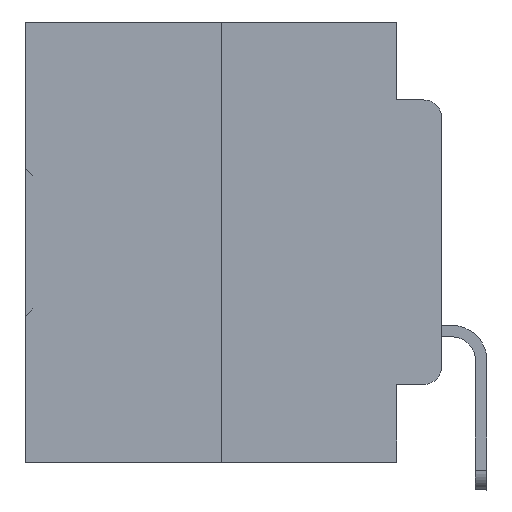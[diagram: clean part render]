
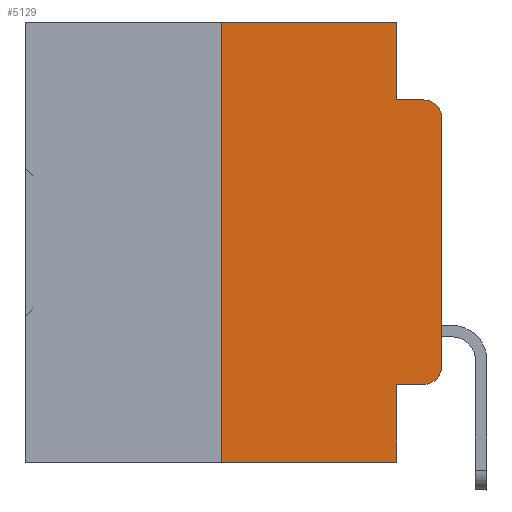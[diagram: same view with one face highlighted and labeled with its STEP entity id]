
A CAD part, left-side view. The second image highlights one B-rep face of the part: STEP entity #5129.
In plain terms, the highlighted planar face has unit normal (-1, 0, 0).
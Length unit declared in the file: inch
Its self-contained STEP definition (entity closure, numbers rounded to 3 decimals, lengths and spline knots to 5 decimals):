
#219 = DIRECTION ( 'NONE',  ( 1., 0., 0. ) ) ;
#1815 = CARTESIAN_POINT ( 'NONE',  ( 0., 0.02, -0.1085 ) ) ;
#3067 = VECTOR ( 'NONE', #6781, 39.37008 ) ;
#3185 = CARTESIAN_POINT ( 'NONE',  ( 0., 0.051, 0. ) ) ;
#3382 = DIRECTION ( 'NONE',  ( 0., 0., 1. ) ) ;
#3490 = CARTESIAN_POINT ( 'NONE',  ( 0., 0.25, 0. ) ) ;
#3536 = CARTESIAN_POINT ( 'NONE',  ( 0., 0., -0.3915 ) ) ;
#4029 = VERTEX_POINT ( 'NONE', #16849 ) ;
#4118 = VERTEX_POINT ( 'NONE', #9675 ) ;
#4264 = AXIS2_PLACEMENT_3D ( 'NONE', #32118, #4676, #4436 ) ;
#4436 = DIRECTION ( 'NONE',  ( 0., 0., -1. ) ) ;
#4676 = DIRECTION ( 'NONE',  ( -1., 0., 0. ) ) ;
#5129 = ADVANCED_FACE ( 'NONE', ( #27398 ), #30025, .F. ) ;
#5293 = EDGE_CURVE ( 'NONE', #20373, #29072, #19749, .T. ) ;
#5730 = DIRECTION ( 'NONE',  ( 0., 0., -1. ) ) ;
#6280 = CARTESIAN_POINT ( 'NONE',  ( 0., 0.051, -0.0885 ) ) ;
#6712 = EDGE_LOOP ( 'NONE', ( #7500, #19162, #9595, #32900, #20562, #15418, #29869, #10594, #18229, #23644 ) ) ;
#6781 = DIRECTION ( 'NONE',  ( 0., 0., 1. ) ) ;
#7350 = EDGE_CURVE ( 'NONE', #29072, #15682, #24922, .T. ) ;
#7380 = LINE ( 'NONE', #12807, #16774 ) ;
#7500 = ORIENTED_EDGE ( 'NONE', *, *, #5293, .T. ) ;
#7527 = DIRECTION ( 'NONE',  ( 0., 0., -1. ) ) ;
#8580 = VERTEX_POINT ( 'NONE', #26436 ) ;
#8662 = AXIS2_PLACEMENT_3D ( 'NONE', #19694, #219, #5730 ) ;
#9595 = ORIENTED_EDGE ( 'NONE', *, *, #26464, .F. ) ;
#9675 = CARTESIAN_POINT ( 'NONE',  ( 0., 0.02, -0.4115 ) ) ;
#9778 = LINE ( 'NONE', #3490, #32808 ) ;
#10130 = EDGE_CURVE ( 'NONE', #34146, #8580, #9778, .T. ) ;
#10342 = EDGE_CURVE ( 'NONE', #8580, #29618, #15295, .T. ) ;
#10594 = ORIENTED_EDGE ( 'NONE', *, *, #12152, .F. ) ;
#11087 = EDGE_CURVE ( 'NONE', #34146, #18029, #22066, .T. ) ;
#11795 = CARTESIAN_POINT ( 'NONE',  ( 0., 0., -0.1085 ) ) ;
#12152 = EDGE_CURVE ( 'NONE', #4029, #18029, #14723, .T. ) ;
#12328 = CARTESIAN_POINT ( 'NONE',  ( 0., 0.051, 0. ) ) ;
#12807 = CARTESIAN_POINT ( 'NONE',  ( 0., 0.051, -0.0885 ) ) ;
#14183 = AXIS2_PLACEMENT_3D ( 'NONE', #1815, #31512, #7527 ) ;
#14251 = VECTOR ( 'NONE', #14429, 39.37008 ) ;
#14429 = DIRECTION ( 'NONE',  ( 0., 0., -1. ) ) ;
#14723 = LINE ( 'NONE', #12328, #28371 ) ;
#14783 = VECTOR ( 'NONE', #18966, 39.37008 ) ;
#14804 = DIRECTION ( 'NONE',  ( 0., -1., 0. ) ) ;
#15295 = LINE ( 'NONE', #20558, #23442 ) ;
#15418 = ORIENTED_EDGE ( 'NONE', *, *, #10130, .F. ) ;
#15483 = EDGE_CURVE ( 'NONE', #4029, #4118, #30434, .T. ) ;
#15682 = VERTEX_POINT ( 'NONE', #31189 ) ;
#16466 = CARTESIAN_POINT ( 'NONE',  ( 0., 0.051, -0.5 ) ) ;
#16774 = VECTOR ( 'NONE', #23657, 39.37008 ) ;
#16849 = CARTESIAN_POINT ( 'NONE',  ( 0., 0.051, -0.4115 ) ) ;
#16979 = CARTESIAN_POINT ( 'NONE',  ( 0., 0.051, 0. ) ) ;
#18029 = VERTEX_POINT ( 'NONE', #16466 ) ;
#18131 = CARTESIAN_POINT ( 'NONE',  ( 0., 0.473, -0.5 ) ) ;
#18229 = ORIENTED_EDGE ( 'NONE', *, *, #15483, .T. ) ;
#18747 = VERTEX_POINT ( 'NONE', #6280 ) ;
#18831 = CARTESIAN_POINT ( 'NONE',  ( 0., 0.051, -0.4115 ) ) ;
#18966 = DIRECTION ( 'NONE',  ( 0., -1., 0. ) ) ;
#19162 = ORIENTED_EDGE ( 'NONE', *, *, #7350, .T. ) ;
#19694 = CARTESIAN_POINT ( 'NONE',  ( 0., 0.473, 0. ) ) ;
#19749 = LINE ( 'NONE', #28594, #3067 ) ;
#19797 = VECTOR ( 'NONE', #32768, 39.37008 ) ;
#20373 = VERTEX_POINT ( 'NONE', #3536 ) ;
#20558 = CARTESIAN_POINT ( 'NONE',  ( 0., 0.473, 0. ) ) ;
#20562 = ORIENTED_EDGE ( 'NONE', *, *, #10342, .F. ) ;
#22066 = LINE ( 'NONE', #18131, #14783 ) ;
#22387 = LINE ( 'NONE', #16979, #14251 ) ;
#23442 = VECTOR ( 'NONE', #14804, 39.37008 ) ;
#23605 = EDGE_CURVE ( 'NONE', #4118, #20373, #24815, .T. ) ;
#23644 = ORIENTED_EDGE ( 'NONE', *, *, #23605, .T. ) ;
#23657 = DIRECTION ( 'NONE',  ( 0., -1., 0. ) ) ;
#24815 = CIRCLE ( 'NONE', #4264, 0.02 ) ;
#24922 = CIRCLE ( 'NONE', #14183, 0.02 ) ;
#26436 = CARTESIAN_POINT ( 'NONE',  ( 0., 0.25, 0. ) ) ;
#26464 = EDGE_CURVE ( 'NONE', #18747, #15682, #7380, .T. ) ;
#27398 = FACE_OUTER_BOUND ( 'NONE', #6712, .T. ) ;
#28371 = VECTOR ( 'NONE', #28652, 39.37008 ) ;
#28594 = CARTESIAN_POINT ( 'NONE',  ( 0., 0., 0. ) ) ;
#28652 = DIRECTION ( 'NONE',  ( 0., 0., -1. ) ) ;
#29072 = VERTEX_POINT ( 'NONE', #11795 ) ;
#29618 = VERTEX_POINT ( 'NONE', #3185 ) ;
#29869 = ORIENTED_EDGE ( 'NONE', *, *, #11087, .T. ) ;
#30025 = PLANE ( 'NONE',  #8662 ) ;
#30434 = LINE ( 'NONE', #18831, #19797 ) ;
#31189 = CARTESIAN_POINT ( 'NONE',  ( 0., 0.02, -0.0885 ) ) ;
#31305 = EDGE_CURVE ( 'NONE', #29618, #18747, #22387, .T. ) ;
#31512 = DIRECTION ( 'NONE',  ( -1., 0., 0. ) ) ;
#32118 = CARTESIAN_POINT ( 'NONE',  ( 0., 0.02, -0.3915 ) ) ;
#32768 = DIRECTION ( 'NONE',  ( 0., -1., 0. ) ) ;
#32808 = VECTOR ( 'NONE', #3382, 39.37008 ) ;
#32900 = ORIENTED_EDGE ( 'NONE', *, *, #31305, .F. ) ;
#33315 = CARTESIAN_POINT ( 'NONE',  ( 0., 0.25, -0.5 ) ) ;
#34146 = VERTEX_POINT ( 'NONE', #33315 ) ;
